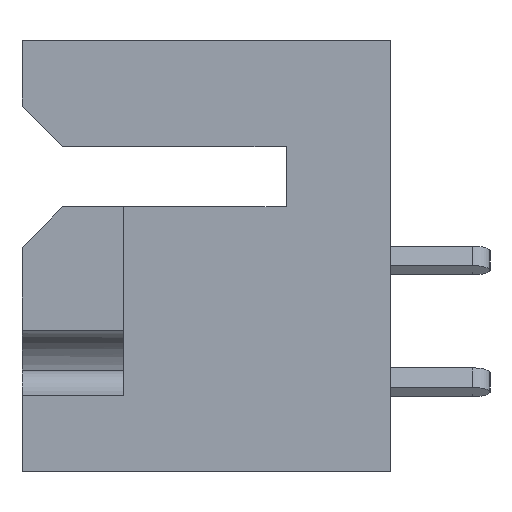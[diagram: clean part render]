
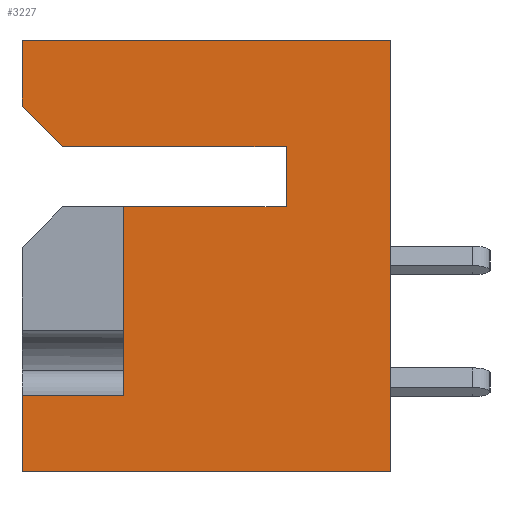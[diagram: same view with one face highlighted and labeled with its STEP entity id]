
A CAD part, left-side view. The second image highlights one B-rep face of the part: STEP entity #3227.
In plain terms, the highlighted planar face has unit normal (-1, 0, 0).
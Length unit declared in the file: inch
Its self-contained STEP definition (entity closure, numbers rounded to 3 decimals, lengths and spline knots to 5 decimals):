
#293 = EDGE_CURVE ( 'NONE', #11397, #4410, #11709, .T. ) ;
#373 = VERTEX_POINT ( 'NONE', #2297 ) ;
#487 = DIRECTION ( 'NONE',  ( 0., 0., -1. ) ) ;
#1227 = LINE ( 'NONE', #16251, #7107 ) ;
#1278 = ORIENTED_EDGE ( 'NONE', *, *, #11260, .F. ) ;
#1370 = EDGE_CURVE ( 'NONE', #4410, #18731, #3485, .T. ) ;
#1659 = CARTESIAN_POINT ( 'NONE',  ( 0., 0.328, -0.205 ) ) ;
#1667 = PLANE ( 'NONE',  #12565 ) ;
#1889 = VERTEX_POINT ( 'NONE', #16840 ) ;
#1999 = VECTOR ( 'NONE', #4553, 39.37008 ) ;
#2016 = LINE ( 'NONE', #4503, #8167 ) ;
#2203 = ORIENTED_EDGE ( 'NONE', *, *, #7482, .F. ) ;
#2212 = DIRECTION ( 'NONE',  ( 0., 1., 0. ) ) ;
#2297 = CARTESIAN_POINT ( 'NONE',  ( 0., 0.453, -0.531 ) ) ;
#2364 = VERTEX_POINT ( 'NONE', #1659 ) ;
#3022 = CARTESIAN_POINT ( 'NONE',  ( 0., 0.128, -0.131 ) ) ;
#3227 = ADVANCED_FACE ( 'NONE', ( #5769 ), #1667, .F. ) ;
#3231 = DIRECTION ( 'NONE',  ( 0., 0., 1. ) ) ;
#3485 = LINE ( 'NONE', #3022, #15296 ) ;
#4061 = ORIENTED_EDGE ( 'NONE', *, *, #18199, .F. ) ;
#4162 = EDGE_LOOP ( 'NONE', ( #9378, #2203, #6149, #18249, #11528, #1278, #8048, #9700, #15539, #10806, #4061 ) ) ;
#4342 = DIRECTION ( 'NONE',  ( 0., 0., 1. ) ) ;
#4410 = VERTEX_POINT ( 'NONE', #7235 ) ;
#4503 = CARTESIAN_POINT ( 'NONE',  ( 0., 0.453, 0. ) ) ;
#4553 = DIRECTION ( 'NONE',  ( 0., -1., 0. ) ) ;
#4958 = DIRECTION ( 'NONE',  ( 1., 0., 0. ) ) ;
#5145 = CARTESIAN_POINT ( 'NONE',  ( 0., 0.128, -0.131 ) ) ;
#5769 = FACE_OUTER_BOUND ( 'NONE', #4162, .T. ) ;
#6149 = ORIENTED_EDGE ( 'NONE', *, *, #14670, .T. ) ;
#6177 = CARTESIAN_POINT ( 'NONE',  ( 0., 0.128, -0.205 ) ) ;
#6234 = CARTESIAN_POINT ( 'NONE',  ( 0., 0.453, 0. ) ) ;
#6263 = DIRECTION ( 'NONE',  ( 0., 0., 1. ) ) ;
#6345 = VECTOR ( 'NONE', #14848, 39.37008 ) ;
#6506 = CARTESIAN_POINT ( 'NONE',  ( 0., 0., 0. ) ) ;
#6927 = EDGE_CURVE ( 'NONE', #20165, #1889, #8427, .T. ) ;
#6981 = CARTESIAN_POINT ( 'NONE',  ( 0., 0.453, -0.081 ) ) ;
#7107 = VECTOR ( 'NONE', #12984, 39.37008 ) ;
#7235 = CARTESIAN_POINT ( 'NONE',  ( 0., 0.128, -0.131 ) ) ;
#7482 = EDGE_CURVE ( 'NONE', #373, #16354, #2016, .T. ) ;
#7501 = LINE ( 'NONE', #10085, #16777 ) ;
#7768 = EDGE_CURVE ( 'NONE', #18416, #1889, #15096, .T. ) ;
#8048 = ORIENTED_EDGE ( 'NONE', *, *, #21337, .T. ) ;
#8135 = LINE ( 'NONE', #9363, #21047 ) ;
#8167 = VECTOR ( 'NONE', #6263, 39.37008 ) ;
#8427 = LINE ( 'NONE', #6506, #18505 ) ;
#8601 = DIRECTION ( 'NONE',  ( 0., -1., 0. ) ) ;
#8691 = VECTOR ( 'NONE', #17189, 39.37008 ) ;
#9363 = CARTESIAN_POINT ( 'NONE',  ( 0., 0.403, -0.131 ) ) ;
#9378 = ORIENTED_EDGE ( 'NONE', *, *, #20517, .T. ) ;
#9700 = ORIENTED_EDGE ( 'NONE', *, *, #1370, .F. ) ;
#10085 = CARTESIAN_POINT ( 'NONE',  ( 0., 0.128, -0.205 ) ) ;
#10203 = CARTESIAN_POINT ( 'NONE',  ( 0., 0., -0.531 ) ) ;
#10806 = ORIENTED_EDGE ( 'NONE', *, *, #15130, .T. ) ;
#11260 = EDGE_CURVE ( 'NONE', #17839, #18416, #12124, .T. ) ;
#11397 = VERTEX_POINT ( 'NONE', #6177 ) ;
#11528 = ORIENTED_EDGE ( 'NONE', *, *, #7768, .F. ) ;
#11709 = LINE ( 'NONE', #5145, #6345 ) ;
#12124 = LINE ( 'NONE', #12493, #20427 ) ;
#12128 = VECTOR ( 'NONE', #8601, 39.37008 ) ;
#12247 = CARTESIAN_POINT ( 'NONE',  ( 0., 0.328, -0.437 ) ) ;
#12412 = LINE ( 'NONE', #15150, #12128 ) ;
#12493 = CARTESIAN_POINT ( 'NONE',  ( 0., 0.453, 0. ) ) ;
#12565 = AXIS2_PLACEMENT_3D ( 'NONE', #13116, #4958, #487 ) ;
#12984 = DIRECTION ( 'NONE',  ( 0., 0., 1. ) ) ;
#13116 = CARTESIAN_POINT ( 'NONE',  ( 0., 0.453, 0. ) ) ;
#13299 = DIRECTION ( 'NONE',  ( 0., 1., 0. ) ) ;
#14234 = DIRECTION ( 'NONE',  ( 0., -0.707, -0.707 ) ) ;
#14576 = CARTESIAN_POINT ( 'NONE',  ( 0., 0.403, -0.131 ) ) ;
#14670 = EDGE_CURVE ( 'NONE', #373, #20165, #12412, .T. ) ;
#14848 = DIRECTION ( 'NONE',  ( 0., 0., 1. ) ) ;
#15096 = LINE ( 'NONE', #6234, #1999 ) ;
#15130 = EDGE_CURVE ( 'NONE', #11397, #2364, #7501, .T. ) ;
#15150 = CARTESIAN_POINT ( 'NONE',  ( 0., 0.453, -0.531 ) ) ;
#15296 = VECTOR ( 'NONE', #2212, 39.37008 ) ;
#15311 = CARTESIAN_POINT ( 'NONE',  ( 0., 0.453, 0. ) ) ;
#15539 = ORIENTED_EDGE ( 'NONE', *, *, #293, .F. ) ;
#16073 = CARTESIAN_POINT ( 'NONE',  ( 0., 0.328, -0.437 ) ) ;
#16251 = CARTESIAN_POINT ( 'NONE',  ( 0., 0.328, -0.205 ) ) ;
#16354 = VERTEX_POINT ( 'NONE', #17980 ) ;
#16777 = VECTOR ( 'NONE', #13299, 39.37008 ) ;
#16840 = CARTESIAN_POINT ( 'NONE',  ( 0., 0., 0. ) ) ;
#17189 = DIRECTION ( 'NONE',  ( 0., 1., 0. ) ) ;
#17467 = VERTEX_POINT ( 'NONE', #16073 ) ;
#17839 = VERTEX_POINT ( 'NONE', #6981 ) ;
#17980 = CARTESIAN_POINT ( 'NONE',  ( 0., 0.453, -0.437 ) ) ;
#18199 = EDGE_CURVE ( 'NONE', #17467, #2364, #1227, .T. ) ;
#18249 = ORIENTED_EDGE ( 'NONE', *, *, #6927, .T. ) ;
#18416 = VERTEX_POINT ( 'NONE', #15311 ) ;
#18505 = VECTOR ( 'NONE', #3231, 39.37008 ) ;
#18731 = VERTEX_POINT ( 'NONE', #14576 ) ;
#19291 = LINE ( 'NONE', #12247, #8691 ) ;
#20165 = VERTEX_POINT ( 'NONE', #10203 ) ;
#20427 = VECTOR ( 'NONE', #4342, 39.37008 ) ;
#20517 = EDGE_CURVE ( 'NONE', #17467, #16354, #19291, .T. ) ;
#21047 = VECTOR ( 'NONE', #14234, 39.37008 ) ;
#21337 = EDGE_CURVE ( 'NONE', #17839, #18731, #8135, .T. ) ;
